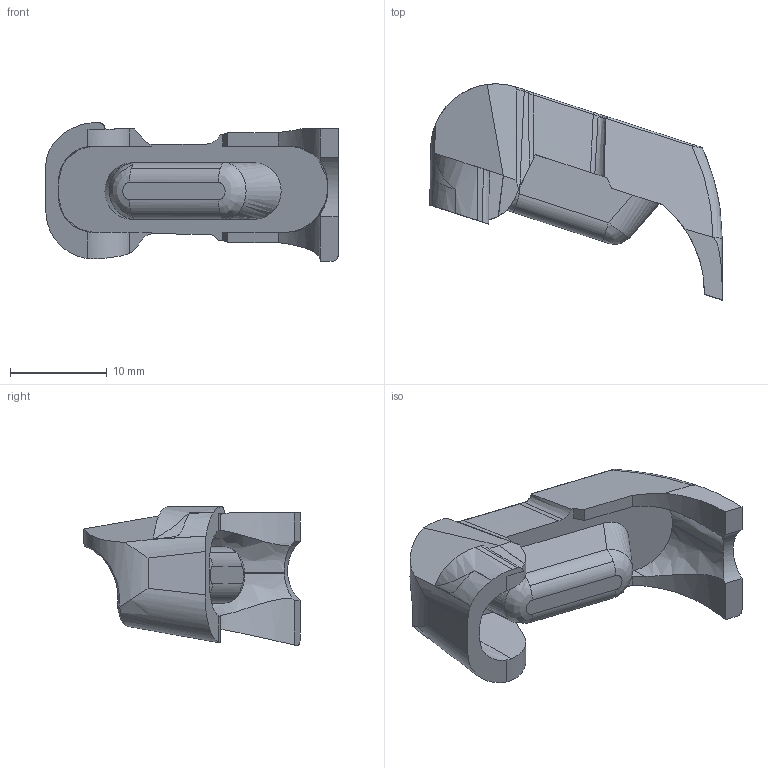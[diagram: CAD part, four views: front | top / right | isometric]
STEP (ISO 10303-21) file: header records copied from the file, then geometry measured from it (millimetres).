
FILE_DESCRIPTION (( 'STEP AP214' ), '1' );
FILE_NAME ('Part31_1.step', '2014-07-30T19:46:24', ( 'WarFairy' ), ( '' ), 'SwSTEP 2.0', 'SolidWorks 2013', '' );
FILE_SCHEMA (( 'AUTOMOTIVE_DESIGN' ));
Length unit declared in the file: millimetre
Products named in the file (1): Part31_1
Bounding box: 30.29 x 22.39 x 14.34 mm (x, y, z)
Volume: 1754 mm3; surface area: 1878.9 mm2
Topology: 1 solids, 1 shells, 108 faces, 278 edges, 172 vertices
Faces by surface type: bspline 61, plane 32, cylinder 15
Entity records: 6188 total; most frequent: CARTESIAN_POINT 4050, ORIENTED_EDGE 554, EDGE_CURVE 277, DIRECTION 235, VERTEX_POINT 172, B_SPLINE_CURVE_WITH_KNOTS 148, EDGE_LOOP 109, FACE_OUTER_BOUND 108
